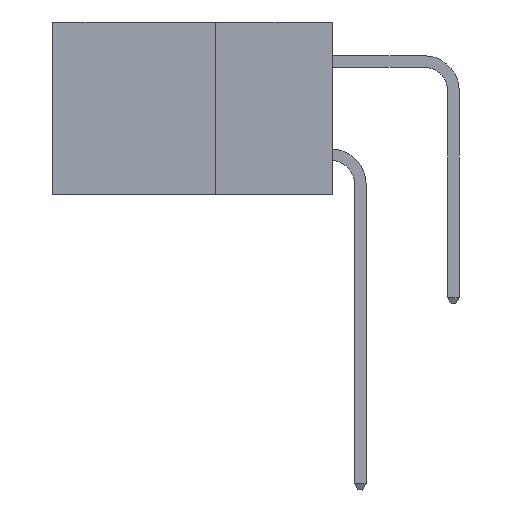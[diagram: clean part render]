
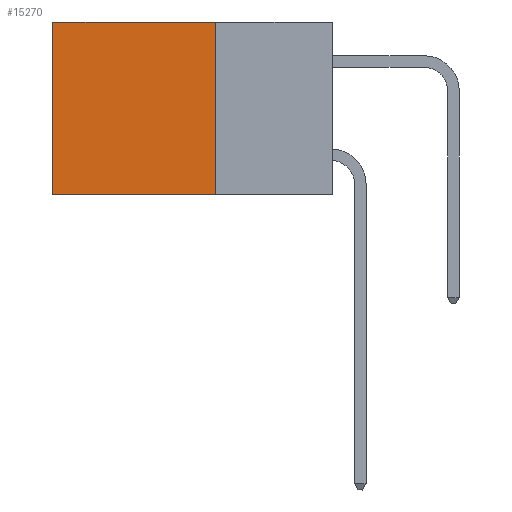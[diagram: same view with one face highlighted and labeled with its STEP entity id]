
A CAD part, left-side view. The second image highlights one B-rep face of the part: STEP entity #15270.
In plain terms, the highlighted planar face has unit normal (-1, 0, 0).
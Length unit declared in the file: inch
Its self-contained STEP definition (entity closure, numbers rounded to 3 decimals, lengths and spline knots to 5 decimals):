
#316 = CARTESIAN_POINT ( 'NONE',  ( 0.298, 0.25, 0. ) ) ;
#1530 = LINE ( 'NONE', #29515, #7400 ) ;
#2514 = CARTESIAN_POINT ( 'NONE',  ( 0.298, 0.25, 0. ) ) ;
#3957 = EDGE_CURVE ( 'NONE', #31897, #17437, #26754, .T. ) ;
#4294 = CARTESIAN_POINT ( 'NONE',  ( 0.298, 0.25, -0.37 ) ) ;
#4450 = LINE ( 'NONE', #4294, #17070 ) ;
#5584 = VERTEX_POINT ( 'NONE', #28976 ) ;
#6462 = CARTESIAN_POINT ( 'NONE',  ( 0.298, 0.25, 0. ) ) ;
#6763 = VECTOR ( 'NONE', #15695, 39.37008 ) ;
#7400 = VECTOR ( 'NONE', #16646, 39.37008 ) ;
#9043 = AXIS2_PLACEMENT_3D ( 'NONE', #2514, #17267, #20079 ) ;
#11134 = VERTEX_POINT ( 'NONE', #25740 ) ;
#14577 = EDGE_LOOP ( 'NONE', ( #25034, #25710, #25983, #22746 ) ) ;
#15270 = ADVANCED_FACE ( 'NONE', ( #25547 ), #32205, .F. ) ;
#15695 = DIRECTION ( 'NONE',  ( 0., 1., 0. ) ) ;
#16290 = CARTESIAN_POINT ( 'NONE',  ( 0.298, 0.6, 0. ) ) ;
#16646 = DIRECTION ( 'NONE',  ( 0., 0., -1. ) ) ;
#16958 = DIRECTION ( 'NONE',  ( 0., 1., 0. ) ) ;
#17070 = VECTOR ( 'NONE', #16958, 39.37008 ) ;
#17267 = DIRECTION ( 'NONE',  ( 1., 0., 0. ) ) ;
#17331 = DIRECTION ( 'NONE',  ( 0., 0., -1. ) ) ;
#17437 = VERTEX_POINT ( 'NONE', #16290 ) ;
#18001 = EDGE_CURVE ( 'NONE', #31897, #11134, #20239, .T. ) ;
#20079 = DIRECTION ( 'NONE',  ( 0., 0., -1. ) ) ;
#20239 = LINE ( 'NONE', #32169, #31921 ) ;
#22746 = ORIENTED_EDGE ( 'NONE', *, *, #3957, .T. ) ;
#22882 = EDGE_CURVE ( 'NONE', #17437, #5584, #1530, .T. ) ;
#25034 = ORIENTED_EDGE ( 'NONE', *, *, #22882, .T. ) ;
#25547 = FACE_OUTER_BOUND ( 'NONE', #14577, .T. ) ;
#25710 = ORIENTED_EDGE ( 'NONE', *, *, #31723, .F. ) ;
#25740 = CARTESIAN_POINT ( 'NONE',  ( 0.298, 0.25, -0.37 ) ) ;
#25983 = ORIENTED_EDGE ( 'NONE', *, *, #18001, .F. ) ;
#26754 = LINE ( 'NONE', #316, #6763 ) ;
#28976 = CARTESIAN_POINT ( 'NONE',  ( 0.298, 0.6, -0.37 ) ) ;
#29515 = CARTESIAN_POINT ( 'NONE',  ( 0.298, 0.6, 0. ) ) ;
#31723 = EDGE_CURVE ( 'NONE', #11134, #5584, #4450, .T. ) ;
#31897 = VERTEX_POINT ( 'NONE', #6462 ) ;
#31921 = VECTOR ( 'NONE', #17331, 39.37008 ) ;
#32169 = CARTESIAN_POINT ( 'NONE',  ( 0.298, 0.25, 0. ) ) ;
#32205 = PLANE ( 'NONE',  #9043 ) ;
